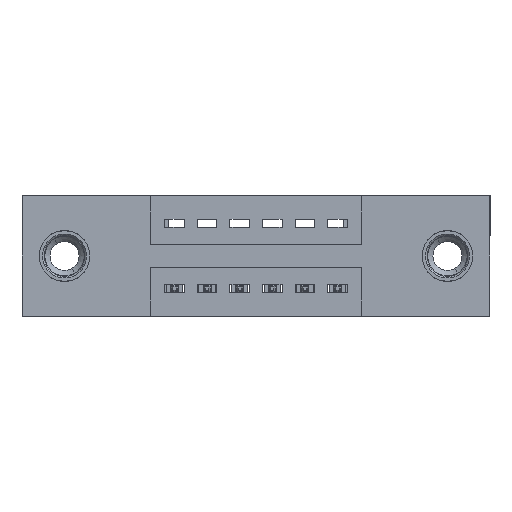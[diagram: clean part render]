
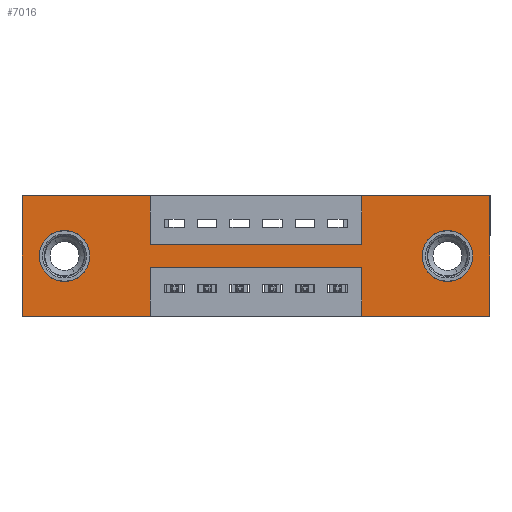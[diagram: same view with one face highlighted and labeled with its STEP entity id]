
A CAD part, front view. The second image highlights one B-rep face of the part: STEP entity #7016.
In plain terms, the highlighted planar face has unit normal (0, -1, 0).
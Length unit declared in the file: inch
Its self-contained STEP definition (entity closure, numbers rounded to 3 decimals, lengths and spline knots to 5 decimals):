
#36 = DIRECTION ( 'NONE',  ( 1., 0., 0. ) ) ;
#229 = VERTEX_POINT ( 'NONE', #10061 ) ;
#336 = VERTEX_POINT ( 'NONE', #7795 ) ;
#383 = CARTESIAN_POINT ( 'NONE',  ( 0.3925, 0., -0.22 ) ) ;
#585 = LINE ( 'NONE', #1788, #651 ) ;
#637 = DIRECTION ( 'NONE',  ( 0., 0., 1. ) ) ;
#651 = VECTOR ( 'NONE', #12464, 39.37008 ) ;
#815 = CARTESIAN_POINT ( 'NONE',  ( 0.13, 0., -0.185 ) ) ;
#828 = DIRECTION ( 'NONE',  ( 0., 0., -1. ) ) ;
#841 = LINE ( 'NONE', #4010, #1710 ) ;
#860 = ORIENTED_EDGE ( 'NONE', *, *, #984, .F. ) ;
#974 = CARTESIAN_POINT ( 'NONE',  ( 0., 0., 0. ) ) ;
#984 = EDGE_CURVE ( 'NONE', #13173, #8193, #13766, .T. ) ;
#986 = VERTEX_POINT ( 'NONE', #7384 ) ;
#1145 = VECTOR ( 'NONE', #4392, 39.37008 ) ;
#1180 = CARTESIAN_POINT ( 'NONE',  ( 0.13, 0., -0.185 ) ) ;
#1598 = VECTOR ( 'NONE', #11317, 39.37008 ) ;
#1710 = VECTOR ( 'NONE', #13917, 39.37008 ) ;
#1719 = LINE ( 'NONE', #5103, #3470 ) ;
#1788 = CARTESIAN_POINT ( 'NONE',  ( 1.435, 0., 0. ) ) ;
#1941 = VERTEX_POINT ( 'NONE', #6170 ) ;
#1965 = EDGE_CURVE ( 'NONE', #2846, #229, #11586, .T. ) ;
#2264 = AXIS2_PLACEMENT_3D ( 'NONE', #10548, #13755, #828 ) ;
#2405 = ORIENTED_EDGE ( 'NONE', *, *, #6467, .F. ) ;
#2418 = LINE ( 'NONE', #12093, #1145 ) ;
#2527 = CARTESIAN_POINT ( 'NONE',  ( 0., 0., -0.37 ) ) ;
#2769 = DIRECTION ( 'NONE',  ( 0., 0., -1. ) ) ;
#2846 = VERTEX_POINT ( 'NONE', #3310 ) ;
#2848 = CARTESIAN_POINT ( 'NONE',  ( 0.3925, 0., 0. ) ) ;
#2933 = CARTESIAN_POINT ( 'NONE',  ( 1.305, 0., -0.263 ) ) ;
#3056 = VECTOR ( 'NONE', #36, 39.37008 ) ;
#3146 = CARTESIAN_POINT ( 'NONE',  ( 0., 0., 0. ) ) ;
#3310 = CARTESIAN_POINT ( 'NONE',  ( 1.0425, 0., -0.37 ) ) ;
#3446 = AXIS2_PLACEMENT_3D ( 'NONE', #815, #5212, #9614 ) ;
#3470 = VECTOR ( 'NONE', #3946, 39.37008 ) ;
#3584 = CARTESIAN_POINT ( 'NONE',  ( 0.3925, 0., -0.22 ) ) ;
#3585 = CARTESIAN_POINT ( 'NONE',  ( 0.3925, 0., 0. ) ) ;
#3625 = FACE_BOUND ( 'NONE', #12822, .T. ) ;
#3636 = ORIENTED_EDGE ( 'NONE', *, *, #7453, .T. ) ;
#3765 = VERTEX_POINT ( 'NONE', #6447 ) ;
#3946 = DIRECTION ( 'NONE',  ( 0., 0., 1. ) ) ;
#4010 = CARTESIAN_POINT ( 'NONE',  ( 0.3925, 0., -0.37 ) ) ;
#4107 = VECTOR ( 'NONE', #6005, 39.37008 ) ;
#4138 = CIRCLE ( 'NONE', #3446, 0.078 ) ;
#4216 = ORIENTED_EDGE ( 'NONE', *, *, #7379, .F. ) ;
#4392 = DIRECTION ( 'NONE',  ( -1., 0., 0. ) ) ;
#4483 = LINE ( 'NONE', #8018, #9906 ) ;
#4586 = AXIS2_PLACEMENT_3D ( 'NONE', #5138, #9545, #8232 ) ;
#4898 = ORIENTED_EDGE ( 'NONE', *, *, #1965, .F. ) ;
#5103 = CARTESIAN_POINT ( 'NONE',  ( 1.0425, 0., 0. ) ) ;
#5138 = CARTESIAN_POINT ( 'NONE',  ( 0., 0., -0.37 ) ) ;
#5150 = EDGE_CURVE ( 'NONE', #7268, #13584, #841, .T. ) ;
#5212 = DIRECTION ( 'NONE',  ( 0., 1., 0. ) ) ;
#6005 = DIRECTION ( 'NONE',  ( 1., 0., 0. ) ) ;
#6048 = CIRCLE ( 'NONE', #8601, 0.078 ) ;
#6140 = DIRECTION ( 'NONE',  ( 0., 0., 1. ) ) ;
#6170 = CARTESIAN_POINT ( 'NONE',  ( 1.0425, 0., 0. ) ) ;
#6201 = EDGE_CURVE ( 'NONE', #9327, #986, #585, .T. ) ;
#6447 = CARTESIAN_POINT ( 'NONE',  ( 0.13, 0., -0.263 ) ) ;
#6467 = EDGE_CURVE ( 'NONE', #8193, #7872, #9079, .T. ) ;
#6542 = ORIENTED_EDGE ( 'NONE', *, *, #9053, .F. ) ;
#6548 = EDGE_CURVE ( 'NONE', #7868, #14033, #9411, .T. ) ;
#6617 = EDGE_CURVE ( 'NONE', #7443, #336, #8485, .T. ) ;
#7016 = ADVANCED_FACE ( 'NONE', ( #13474, #3625, #8028 ), #12411, .T. ) ;
#7116 = AXIS2_PLACEMENT_3D ( 'NONE', #13600, #12535, #8158 ) ;
#7143 = EDGE_LOOP ( 'NONE', ( #11196, #12248, #4898, #4216, #12737, #9503, #6542, #2405, #860, #10016, #7460, #11639 ) ) ;
#7268 = VERTEX_POINT ( 'NONE', #383 ) ;
#7379 = EDGE_CURVE ( 'NONE', #986, #2846, #10181, .T. ) ;
#7384 = CARTESIAN_POINT ( 'NONE',  ( 1.435, 0., -0.37 ) ) ;
#7443 = VERTEX_POINT ( 'NONE', #2933 ) ;
#7453 = EDGE_CURVE ( 'NONE', #336, #7443, #11480, .T. ) ;
#7460 = ORIENTED_EDGE ( 'NONE', *, *, #6548, .F. ) ;
#7539 = ORIENTED_EDGE ( 'NONE', *, *, #8209, .T. ) ;
#7795 = CARTESIAN_POINT ( 'NONE',  ( 1.305, 0., -0.107 ) ) ;
#7868 = VERTEX_POINT ( 'NONE', #13181 ) ;
#7872 = VERTEX_POINT ( 'NONE', #10973 ) ;
#7918 = EDGE_LOOP ( 'NONE', ( #3636, #9686 ) ) ;
#8018 = CARTESIAN_POINT ( 'NONE',  ( 0., 0., 0. ) ) ;
#8028 = FACE_OUTER_BOUND ( 'NONE', #7143, .T. ) ;
#8044 = CARTESIAN_POINT ( 'NONE',  ( 0.3925, 0., -0.15 ) ) ;
#8158 = DIRECTION ( 'NONE',  ( 0., 0., -1. ) ) ;
#8193 = VERTEX_POINT ( 'NONE', #10407 ) ;
#8209 = EDGE_CURVE ( 'NONE', #12147, #3765, #4138, .T. ) ;
#8232 = DIRECTION ( 'NONE',  ( 0., 0., -1. ) ) ;
#8485 = CIRCLE ( 'NONE', #2264, 0.078 ) ;
#8497 = EDGE_CURVE ( 'NONE', #1941, #9327, #4483, .T. ) ;
#8601 = AXIS2_PLACEMENT_3D ( 'NONE', #1180, #14133, #12059 ) ;
#8893 = DIRECTION ( 'NONE',  ( 1., 0., 0. ) ) ;
#9053 = EDGE_CURVE ( 'NONE', #7872, #1941, #1719, .T. ) ;
#9079 = LINE ( 'NONE', #8044, #4107 ) ;
#9327 = VERTEX_POINT ( 'NONE', #10149 ) ;
#9340 = EDGE_CURVE ( 'NONE', #229, #7268, #9932, .T. ) ;
#9411 = LINE ( 'NONE', #13694, #11691 ) ;
#9503 = ORIENTED_EDGE ( 'NONE', *, *, #8497, .F. ) ;
#9545 = DIRECTION ( 'NONE',  ( 0., -1., 0. ) ) ;
#9614 = DIRECTION ( 'NONE',  ( 0., 0., 1. ) ) ;
#9686 = ORIENTED_EDGE ( 'NONE', *, *, #6617, .T. ) ;
#9894 = EDGE_CURVE ( 'NONE', #13584, #7868, #2418, .T. ) ;
#9906 = VECTOR ( 'NONE', #8893, 39.37008 ) ;
#9932 = LINE ( 'NONE', #3584, #11267 ) ;
#10016 = ORIENTED_EDGE ( 'NONE', *, *, #13427, .F. ) ;
#10061 = CARTESIAN_POINT ( 'NONE',  ( 1.0425, 0., -0.22 ) ) ;
#10149 = CARTESIAN_POINT ( 'NONE',  ( 1.435, 0., 0. ) ) ;
#10181 = LINE ( 'NONE', #2527, #1598 ) ;
#10382 = CARTESIAN_POINT ( 'NONE',  ( 1.0425, 0., -0.37 ) ) ;
#10407 = CARTESIAN_POINT ( 'NONE',  ( 0.3925, 0., -0.15 ) ) ;
#10548 = CARTESIAN_POINT ( 'NONE',  ( 1.305, 0., -0.185 ) ) ;
#10973 = CARTESIAN_POINT ( 'NONE',  ( 1.0425, 0., -0.15 ) ) ;
#11196 = ORIENTED_EDGE ( 'NONE', *, *, #5150, .F. ) ;
#11267 = VECTOR ( 'NONE', #12364, 39.37008 ) ;
#11317 = DIRECTION ( 'NONE',  ( -1., 0., 0. ) ) ;
#11480 = CIRCLE ( 'NONE', #7116, 0.078 ) ;
#11586 = LINE ( 'NONE', #10382, #13125 ) ;
#11639 = ORIENTED_EDGE ( 'NONE', *, *, #9894, .F. ) ;
#11691 = VECTOR ( 'NONE', #6140, 39.37008 ) ;
#11963 = ORIENTED_EDGE ( 'NONE', *, *, #13457, .T. ) ;
#11991 = VECTOR ( 'NONE', #2769, 39.37008 ) ;
#12059 = DIRECTION ( 'NONE',  ( 0., 0., 1. ) ) ;
#12093 = CARTESIAN_POINT ( 'NONE',  ( 0., 0., -0.37 ) ) ;
#12147 = VERTEX_POINT ( 'NONE', #13089 ) ;
#12248 = ORIENTED_EDGE ( 'NONE', *, *, #9340, .F. ) ;
#12364 = DIRECTION ( 'NONE',  ( -1., 0., 0. ) ) ;
#12411 = PLANE ( 'NONE',  #4586 ) ;
#12464 = DIRECTION ( 'NONE',  ( 0., 0., -1. ) ) ;
#12535 = DIRECTION ( 'NONE',  ( 0., 1., 0. ) ) ;
#12737 = ORIENTED_EDGE ( 'NONE', *, *, #6201, .F. ) ;
#12822 = EDGE_LOOP ( 'NONE', ( #7539, #11963 ) ) ;
#13089 = CARTESIAN_POINT ( 'NONE',  ( 0.13, 0., -0.107 ) ) ;
#13125 = VECTOR ( 'NONE', #637, 39.37008 ) ;
#13173 = VERTEX_POINT ( 'NONE', #3585 ) ;
#13181 = CARTESIAN_POINT ( 'NONE',  ( 0., 0., -0.37 ) ) ;
#13427 = EDGE_CURVE ( 'NONE', #14033, #13173, #14060, .T. ) ;
#13457 = EDGE_CURVE ( 'NONE', #3765, #12147, #6048, .T. ) ;
#13474 = FACE_BOUND ( 'NONE', #7918, .T. ) ;
#13484 = CARTESIAN_POINT ( 'NONE',  ( 0.3925, 0., -0.37 ) ) ;
#13584 = VERTEX_POINT ( 'NONE', #13484 ) ;
#13600 = CARTESIAN_POINT ( 'NONE',  ( 1.305, 0., -0.185 ) ) ;
#13694 = CARTESIAN_POINT ( 'NONE',  ( 0., 0., 0. ) ) ;
#13755 = DIRECTION ( 'NONE',  ( 0., 1., 0. ) ) ;
#13766 = LINE ( 'NONE', #2848, #11991 ) ;
#13917 = DIRECTION ( 'NONE',  ( 0., 0., -1. ) ) ;
#14033 = VERTEX_POINT ( 'NONE', #3146 ) ;
#14060 = LINE ( 'NONE', #974, #3056 ) ;
#14133 = DIRECTION ( 'NONE',  ( 0., 1., 0. ) ) ;
